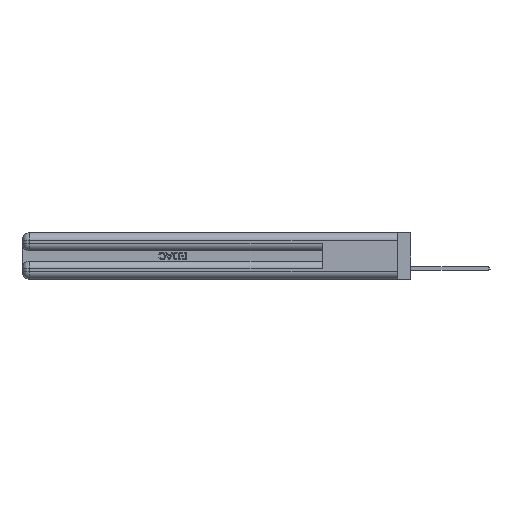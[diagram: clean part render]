
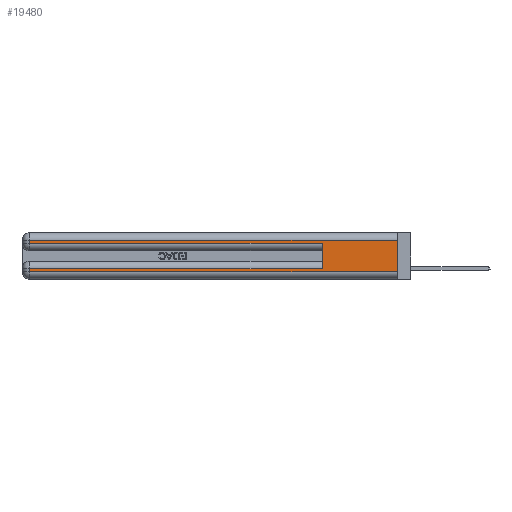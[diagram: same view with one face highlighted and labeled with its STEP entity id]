
A CAD part, left-side view. The second image highlights one B-rep face of the part: STEP entity #19480.
In plain terms, the highlighted planar face has unit normal (-1, 0, 0).
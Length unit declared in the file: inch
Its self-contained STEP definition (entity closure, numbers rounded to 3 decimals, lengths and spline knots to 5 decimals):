
#2072 = EDGE_CURVE ( 'NONE', #32157, #43027, #44307, .T. ) ;
#2503 = VERTEX_POINT ( 'NONE', #21098 ) ;
#3487 = VERTEX_POINT ( 'NONE', #41564 ) ;
#5437 = VECTOR ( 'NONE', #17167, 39.37008 ) ;
#6600 = VERTEX_POINT ( 'NONE', #32286 ) ;
#6945 = DIRECTION ( 'NONE',  ( 0., -1., 0. ) ) ;
#7424 = ORIENTED_EDGE ( 'NONE', *, *, #41607, .T. ) ;
#8034 = DIRECTION ( 'NONE',  ( 0., 0., -1. ) ) ;
#8457 = CARTESIAN_POINT ( 'NONE',  ( 0., 0., 0.285 ) ) ;
#8631 = EDGE_CURVE ( 'NONE', #2503, #39572, #21845, .T. ) ;
#9549 = DIRECTION ( 'NONE',  ( 0., 1., 0. ) ) ;
#9636 = VECTOR ( 'NONE', #22891, 39.37008 ) ;
#10793 = CARTESIAN_POINT ( 'NONE',  ( 0., 2.94, 0.085 ) ) ;
#10886 = CARTESIAN_POINT ( 'NONE',  ( 0., 0., 0.06 ) ) ;
#12115 = EDGE_CURVE ( 'NONE', #29938, #2503, #20356, .T. ) ;
#12286 = CARTESIAN_POINT ( 'NONE',  ( 0., 0., 0.37 ) ) ;
#12543 = CARTESIAN_POINT ( 'NONE',  ( 0., 0.6, 0.085 ) ) ;
#13262 = ORIENTED_EDGE ( 'NONE', *, *, #30261, .F. ) ;
#15270 = CARTESIAN_POINT ( 'NONE',  ( 0., 0.6, 0.285 ) ) ;
#15737 = AXIS2_PLACEMENT_3D ( 'NONE', #12286, #38218, #8034 ) ;
#16520 = CARTESIAN_POINT ( 'NONE',  ( 0., 0., 0.31 ) ) ;
#17167 = DIRECTION ( 'NONE',  ( 0., 1., 0. ) ) ;
#17325 = CARTESIAN_POINT ( 'NONE',  ( 0., 0., 0.085 ) ) ;
#17947 = CARTESIAN_POINT ( 'NONE',  ( 0., 2.94, 0.37 ) ) ;
#18781 = CARTESIAN_POINT ( 'NONE',  ( 0., 0.6, 0.145 ) ) ;
#19480 = ADVANCED_FACE ( 'NONE', ( #26431 ), #23308, .F. ) ;
#20356 = LINE ( 'NONE', #35112, #47040 ) ;
#21098 = CARTESIAN_POINT ( 'NONE',  ( 0., 2.94, 0.285 ) ) ;
#21768 = VECTOR ( 'NONE', #9549, 39.37008 ) ;
#21845 = LINE ( 'NONE', #8457, #35245 ) ;
#22159 = LINE ( 'NONE', #18781, #38428 ) ;
#22891 = DIRECTION ( 'NONE',  ( 0., 0., -1. ) ) ;
#23308 = PLANE ( 'NONE',  #15737 ) ;
#23469 = CARTESIAN_POINT ( 'NONE',  ( 0., 2.94, 0.31 ) ) ;
#26431 = FACE_OUTER_BOUND ( 'NONE', #43566, .T. ) ;
#28618 = EDGE_CURVE ( 'NONE', #3487, #41008, #31284, .T. ) ;
#29112 = ORIENTED_EDGE ( 'NONE', *, *, #2072, .T. ) ;
#29463 = DIRECTION ( 'NONE',  ( 0., 0., -1. ) ) ;
#29938 = VERTEX_POINT ( 'NONE', #23469 ) ;
#30017 = DIRECTION ( 'NONE',  ( 0., 0., 1. ) ) ;
#30261 = EDGE_CURVE ( 'NONE', #6600, #41008, #33399, .T. ) ;
#31284 = LINE ( 'NONE', #10886, #34737 ) ;
#31712 = DIRECTION ( 'NONE',  ( 0., -1., 0. ) ) ;
#32157 = VERTEX_POINT ( 'NONE', #12543 ) ;
#32286 = CARTESIAN_POINT ( 'NONE',  ( 0., 0., 0.31 ) ) ;
#33399 = LINE ( 'NONE', #44612, #9636 ) ;
#34415 = ORIENTED_EDGE ( 'NONE', *, *, #8631, .T. ) ;
#34737 = VECTOR ( 'NONE', #6945, 39.37008 ) ;
#35112 = CARTESIAN_POINT ( 'NONE',  ( 0., 2.94, 0.37 ) ) ;
#35201 = ORIENTED_EDGE ( 'NONE', *, *, #46533, .T. ) ;
#35245 = VECTOR ( 'NONE', #31712, 39.37008 ) ;
#35843 = ORIENTED_EDGE ( 'NONE', *, *, #28618, .T. ) ;
#38218 = DIRECTION ( 'NONE',  ( 1., 0., 0. ) ) ;
#38428 = VECTOR ( 'NONE', #30017, 39.37008 ) ;
#39572 = VERTEX_POINT ( 'NONE', #15270 ) ;
#41008 = VERTEX_POINT ( 'NONE', #47346 ) ;
#41435 = LINE ( 'NONE', #16520, #21768 ) ;
#41564 = CARTESIAN_POINT ( 'NONE',  ( 0., 2.94, 0.06 ) ) ;
#41607 = EDGE_CURVE ( 'NONE', #43027, #3487, #46563, .T. ) ;
#42561 = EDGE_CURVE ( 'NONE', #32157, #39572, #22159, .T. ) ;
#42775 = ORIENTED_EDGE ( 'NONE', *, *, #42561, .F. ) ;
#42999 = DIRECTION ( 'NONE',  ( 0., 0., -1. ) ) ;
#43027 = VERTEX_POINT ( 'NONE', #10793 ) ;
#43566 = EDGE_LOOP ( 'NONE', ( #13262, #35201, #46222, #34415, #42775, #29112, #7424, #35843 ) ) ;
#44307 = LINE ( 'NONE', #17325, #5437 ) ;
#44612 = CARTESIAN_POINT ( 'NONE',  ( 0., 0., 0.37 ) ) ;
#45348 = VECTOR ( 'NONE', #29463, 39.37008 ) ;
#46222 = ORIENTED_EDGE ( 'NONE', *, *, #12115, .T. ) ;
#46533 = EDGE_CURVE ( 'NONE', #6600, #29938, #41435, .T. ) ;
#46563 = LINE ( 'NONE', #17947, #45348 ) ;
#47040 = VECTOR ( 'NONE', #42999, 39.37008 ) ;
#47346 = CARTESIAN_POINT ( 'NONE',  ( 0., 0., 0.06 ) ) ;
